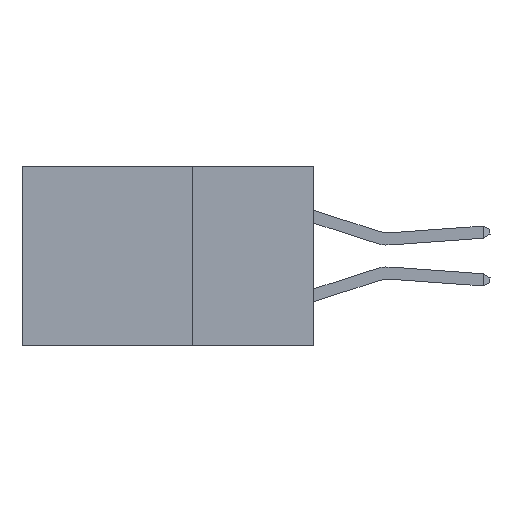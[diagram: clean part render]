
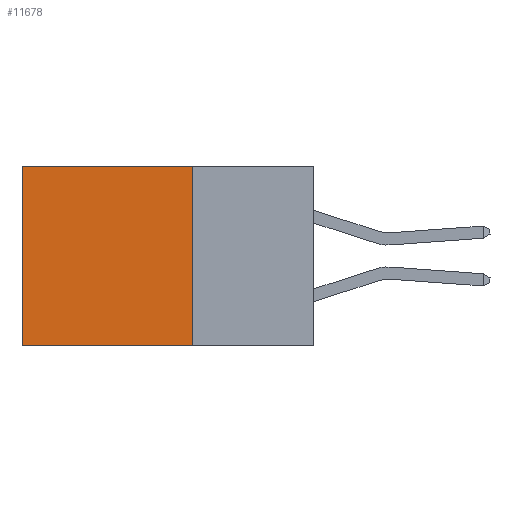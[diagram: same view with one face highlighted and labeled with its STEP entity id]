
A CAD part, left-side view. The second image highlights one B-rep face of the part: STEP entity #11678.
In plain terms, the highlighted planar face has unit normal (-1, 0, 0).
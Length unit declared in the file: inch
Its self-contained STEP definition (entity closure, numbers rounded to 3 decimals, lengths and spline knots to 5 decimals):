
#122 = VECTOR ( 'NONE', #15473, 39.37008 ) ;
#347 = ORIENTED_EDGE ( 'NONE', *, *, #6487, .F. ) ;
#943 = LINE ( 'NONE', #17021, #122 ) ;
#1537 = VECTOR ( 'NONE', #1653, 39.37008 ) ;
#1619 = LINE ( 'NONE', #14958, #7749 ) ;
#1653 = DIRECTION ( 'NONE',  ( 0., 1., 0. ) ) ;
#2028 = DIRECTION ( 'NONE',  ( 0., 0., -1. ) ) ;
#2763 = EDGE_CURVE ( 'NONE', #7772, #8639, #943, .T. ) ;
#2849 = EDGE_CURVE ( 'NONE', #3706, #15803, #13128, .T. ) ;
#2851 = CARTESIAN_POINT ( 'NONE',  ( 0.2875, 0.25, 0. ) ) ;
#3706 = VERTEX_POINT ( 'NONE', #13958 ) ;
#4366 = CARTESIAN_POINT ( 'NONE',  ( 0.2875, 0.25, -0.37 ) ) ;
#4684 = PLANE ( 'NONE',  #7425 ) ;
#5565 = VECTOR ( 'NONE', #8719, 39.37008 ) ;
#6487 = EDGE_CURVE ( 'NONE', #7772, #3706, #9515, .T. ) ;
#7425 = AXIS2_PLACEMENT_3D ( 'NONE', #8846, #9960, #2028 ) ;
#7749 = VECTOR ( 'NONE', #8039, 39.37008 ) ;
#7772 = VERTEX_POINT ( 'NONE', #2851 ) ;
#8039 = DIRECTION ( 'NONE',  ( 0., 0., -1. ) ) ;
#8639 = VERTEX_POINT ( 'NONE', #10916 ) ;
#8719 = DIRECTION ( 'NONE',  ( 0., 0., -1. ) ) ;
#8846 = CARTESIAN_POINT ( 'NONE',  ( 0.2875, 0.25, 0. ) ) ;
#8983 = ORIENTED_EDGE ( 'NONE', *, *, #2849, .F. ) ;
#9515 = LINE ( 'NONE', #14206, #5565 ) ;
#9960 = DIRECTION ( 'NONE',  ( 1., 0., 0. ) ) ;
#10051 = EDGE_LOOP ( 'NONE', ( #13994, #8983, #347, #13236 ) ) ;
#10916 = CARTESIAN_POINT ( 'NONE',  ( 0.2875, 0.6, 0. ) ) ;
#11678 = ADVANCED_FACE ( 'NONE', ( #15232 ), #4684, .F. ) ;
#13128 = LINE ( 'NONE', #4366, #1537 ) ;
#13236 = ORIENTED_EDGE ( 'NONE', *, *, #2763, .T. ) ;
#13958 = CARTESIAN_POINT ( 'NONE',  ( 0.2875, 0.25, -0.37 ) ) ;
#13994 = ORIENTED_EDGE ( 'NONE', *, *, #14872, .T. ) ;
#14206 = CARTESIAN_POINT ( 'NONE',  ( 0.2875, 0.25, 0. ) ) ;
#14872 = EDGE_CURVE ( 'NONE', #8639, #15803, #1619, .T. ) ;
#14958 = CARTESIAN_POINT ( 'NONE',  ( 0.2875, 0.6, 0. ) ) ;
#15020 = CARTESIAN_POINT ( 'NONE',  ( 0.2875, 0.6, -0.37 ) ) ;
#15232 = FACE_OUTER_BOUND ( 'NONE', #10051, .T. ) ;
#15473 = DIRECTION ( 'NONE',  ( 0., 1., 0. ) ) ;
#15803 = VERTEX_POINT ( 'NONE', #15020 ) ;
#17021 = CARTESIAN_POINT ( 'NONE',  ( 0.2875, 0.25, 0. ) ) ;
